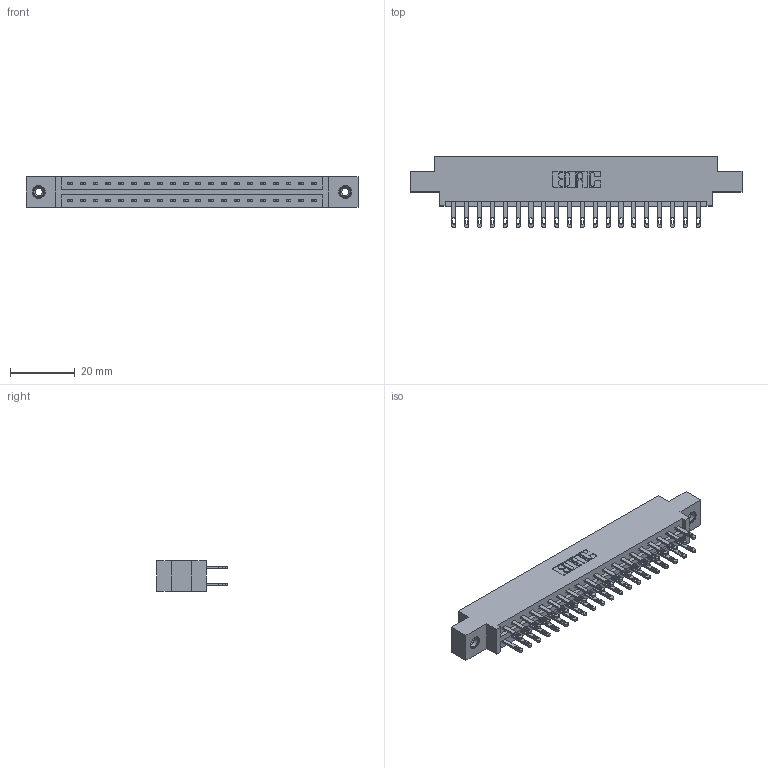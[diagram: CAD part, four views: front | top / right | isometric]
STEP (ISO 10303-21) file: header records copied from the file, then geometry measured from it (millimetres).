
FILE_DESCRIPTION (( 'STEP AP203' ), '1' );
FILE_NAME ('337-040-500-808.STEP', '2018-08-08T08:50:08', ( '' ), ( '' ), 'SwSTEP 2.0', 'SolidWorks 2016', '' );
FILE_SCHEMA (( 'CONFIG_CONTROL_DESIGN' ));
Length unit declared in the file: inch
Products named in the file (4): 345-292-001_345-293-100; 345-250-001_345-250-003-102; 337-040-500-808; 337 Part_0.170 Offset - 0.156 Dia-TI
Assembly tree (43 placements, depth 2):
  337-040-500-808
    337 Part_0.170 Offset - 0.156 Dia-TI
    345-292-001_345-293-100  x40
    345-250-001_345-250-003-102  x2
Bounding box: 102.26 x 21.85 x 9.4 mm (x, y, z)
Volume: 10482.4 mm3; surface area: 12212.2 mm2
Topology: 43 solids, 43 shells, 2178 faces, 6579 edges, 4378 vertices
Faces by surface type: plane 1386, cylinder 776, cone 12, torus 4
Entity records: 19600 total; most frequent: CARTESIAN_POINT 3301, ORIENTED_EDGE 3230, DIRECTION 2881, EDGE_CURVE 1615, LINE 1463, VECTOR 1463, VERTEX_POINT 1072, AXIS2_PLACEMENT_3D 709
